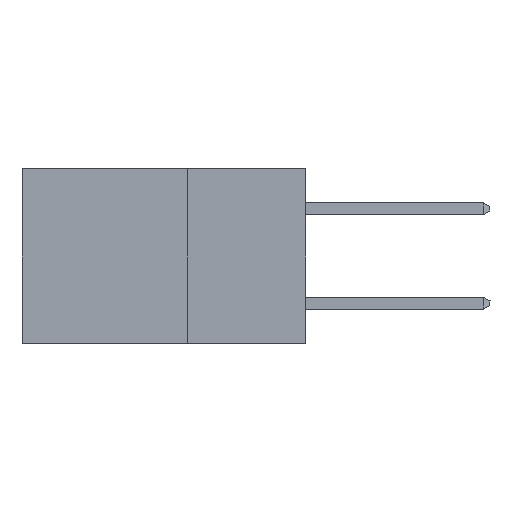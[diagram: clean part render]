
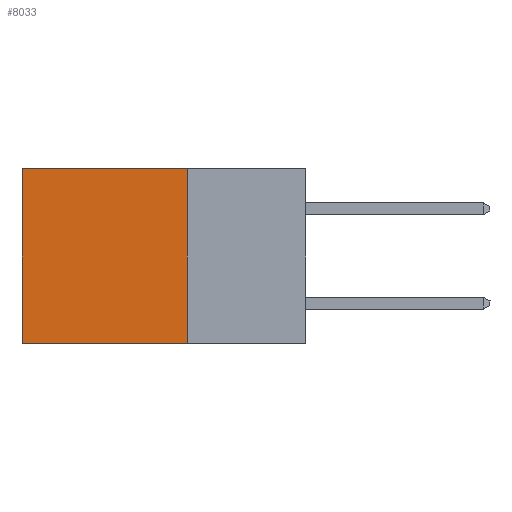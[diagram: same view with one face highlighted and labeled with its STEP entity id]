
A CAD part, left-side view. The second image highlights one B-rep face of the part: STEP entity #8033.
In plain terms, the highlighted planar face has unit normal (-1, 0, 0).
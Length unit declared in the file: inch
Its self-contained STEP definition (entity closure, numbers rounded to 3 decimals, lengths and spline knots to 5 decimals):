
#1371 = VECTOR ( 'NONE', #4498, 39.37008 ) ;
#1394 = ORIENTED_EDGE ( 'NONE', *, *, #3624, .T. ) ;
#1709 = CARTESIAN_POINT ( 'NONE',  ( 0.2615, 0.25, 0. ) ) ;
#1728 = CARTESIAN_POINT ( 'NONE',  ( 0.2615, 0.25, 0. ) ) ;
#2246 = LINE ( 'NONE', #4672, #1371 ) ;
#2625 = ORIENTED_EDGE ( 'NONE', *, *, #4767, .F. ) ;
#3624 = EDGE_CURVE ( 'NONE', #6122, #5844, #2246, .T. ) ;
#4382 = VECTOR ( 'NONE', #5368, 39.37008 ) ;
#4498 = DIRECTION ( 'NONE',  ( 0., 0., -1. ) ) ;
#4672 = CARTESIAN_POINT ( 'NONE',  ( 0.2615, 0.6, -0.37 ) ) ;
#4767 = EDGE_CURVE ( 'NONE', #12561, #16146, #6750, .T. ) ;
#5368 = DIRECTION ( 'NONE',  ( 0., 1., 0. ) ) ;
#5415 = CARTESIAN_POINT ( 'NONE',  ( 0.2615, 0.25, -0.37 ) ) ;
#5844 = VERTEX_POINT ( 'NONE', #9788 ) ;
#6122 = VERTEX_POINT ( 'NONE', #9590 ) ;
#6718 = DIRECTION ( 'NONE',  ( 0., 0., -1. ) ) ;
#6750 = LINE ( 'NONE', #6772, #13488 ) ;
#6772 = CARTESIAN_POINT ( 'NONE',  ( 0.2615, 0.25, -0.37 ) ) ;
#8033 = ADVANCED_FACE ( 'NONE', ( #14186 ), #9456, .F. ) ;
#8450 = AXIS2_PLACEMENT_3D ( 'NONE', #9560, #9418, #9402 ) ;
#8738 = LINE ( 'NONE', #1728, #12118 ) ;
#9269 = EDGE_LOOP ( 'NONE', ( #1394, #9823, #2625, #14429 ) ) ;
#9402 = DIRECTION ( 'NONE',  ( 0., 0., -1. ) ) ;
#9418 = DIRECTION ( 'NONE',  ( 1., 0., 0. ) ) ;
#9456 = PLANE ( 'NONE',  #8450 ) ;
#9560 = CARTESIAN_POINT ( 'NONE',  ( 0.2615, 0.25, -0.37 ) ) ;
#9590 = CARTESIAN_POINT ( 'NONE',  ( 0.2615, 0.6, 0. ) ) ;
#9788 = CARTESIAN_POINT ( 'NONE',  ( 0.2615, 0.6, -0.37 ) ) ;
#9823 = ORIENTED_EDGE ( 'NONE', *, *, #11484, .F. ) ;
#11340 = DIRECTION ( 'NONE',  ( 0., 1., 0. ) ) ;
#11484 = EDGE_CURVE ( 'NONE', #16146, #5844, #14482, .T. ) ;
#12118 = VECTOR ( 'NONE', #11340, 39.37008 ) ;
#12561 = VERTEX_POINT ( 'NONE', #1709 ) ;
#13488 = VECTOR ( 'NONE', #6718, 39.37008 ) ;
#14186 = FACE_OUTER_BOUND ( 'NONE', #9269, .T. ) ;
#14429 = ORIENTED_EDGE ( 'NONE', *, *, #14844, .T. ) ;
#14482 = LINE ( 'NONE', #5415, #4382 ) ;
#14601 = CARTESIAN_POINT ( 'NONE',  ( 0.2615, 0.25, -0.37 ) ) ;
#14844 = EDGE_CURVE ( 'NONE', #12561, #6122, #8738, .T. ) ;
#16146 = VERTEX_POINT ( 'NONE', #14601 ) ;
